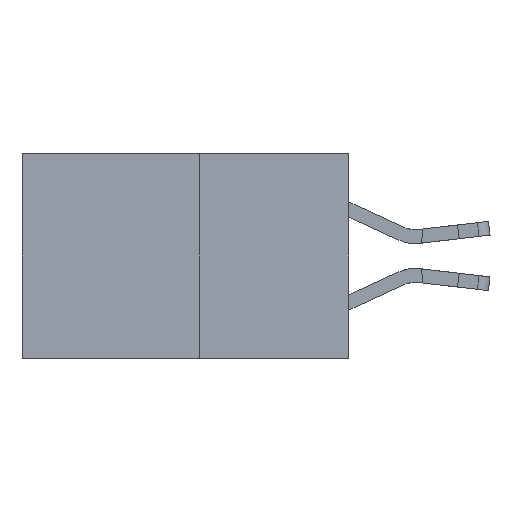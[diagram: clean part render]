
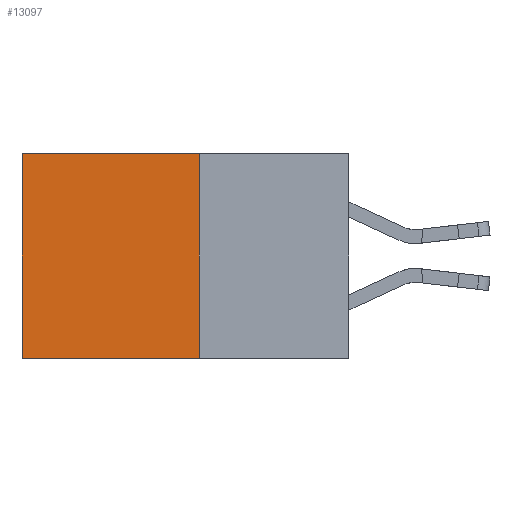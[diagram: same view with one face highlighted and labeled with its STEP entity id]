
A CAD part, left-side view. The second image highlights one B-rep face of the part: STEP entity #13097.
In plain terms, the highlighted planar face has unit normal (-1, 0, 0).
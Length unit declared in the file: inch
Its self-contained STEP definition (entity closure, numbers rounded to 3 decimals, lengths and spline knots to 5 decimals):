
#431 = DIRECTION ( 'NONE',  ( 0., 0., -1. ) ) ;
#689 = EDGE_LOOP ( 'NONE', ( #3078, #10566, #5429, #3585 ) ) ;
#1129 = CARTESIAN_POINT ( 'NONE',  ( 0.277, 0.27, -0.37 ) ) ;
#1178 = EDGE_CURVE ( 'NONE', #10674, #6368, #12203, .T. ) ;
#2004 = CARTESIAN_POINT ( 'NONE',  ( 0.277, 0.59, -0.37 ) ) ;
#2106 = DIRECTION ( 'NONE',  ( 0., 1., 0. ) ) ;
#2155 = LINE ( 'NONE', #2004, #4682 ) ;
#2842 = AXIS2_PLACEMENT_3D ( 'NONE', #1129, #12595, #6492 ) ;
#3014 = CARTESIAN_POINT ( 'NONE',  ( 0.277, 0.27, -0.37 ) ) ;
#3078 = ORIENTED_EDGE ( 'NONE', *, *, #10289, .T. ) ;
#3348 = PLANE ( 'NONE',  #2842 ) ;
#3585 = ORIENTED_EDGE ( 'NONE', *, *, #1178, .T. ) ;
#3649 = VERTEX_POINT ( 'NONE', #10205 ) ;
#4003 = VECTOR ( 'NONE', #6234, 39.37008 ) ;
#4246 = FACE_OUTER_BOUND ( 'NONE', #689, .T. ) ;
#4682 = VECTOR ( 'NONE', #13278, 39.37008 ) ;
#4811 = CARTESIAN_POINT ( 'NONE',  ( 0.277, 0.27, 0. ) ) ;
#5087 = VERTEX_POINT ( 'NONE', #10917 ) ;
#5429 = ORIENTED_EDGE ( 'NONE', *, *, #5829, .F. ) ;
#5443 = EDGE_CURVE ( 'NONE', #5087, #3649, #7518, .T. ) ;
#5736 = LINE ( 'NONE', #8645, #10895 ) ;
#5829 = EDGE_CURVE ( 'NONE', #10674, #5087, #5736, .T. ) ;
#6234 = DIRECTION ( 'NONE',  ( 0., 1., 0. ) ) ;
#6368 = VERTEX_POINT ( 'NONE', #8462 ) ;
#6492 = DIRECTION ( 'NONE',  ( 0., 0., -1. ) ) ;
#7344 = CARTESIAN_POINT ( 'NONE',  ( 0.277, 0.27, 0. ) ) ;
#7518 = LINE ( 'NONE', #3014, #12601 ) ;
#8462 = CARTESIAN_POINT ( 'NONE',  ( 0.277, 0.59, 0. ) ) ;
#8645 = CARTESIAN_POINT ( 'NONE',  ( 0.277, 0.27, -0.37 ) ) ;
#10205 = CARTESIAN_POINT ( 'NONE',  ( 0.277, 0.59, -0.37 ) ) ;
#10289 = EDGE_CURVE ( 'NONE', #6368, #3649, #2155, .T. ) ;
#10566 = ORIENTED_EDGE ( 'NONE', *, *, #5443, .F. ) ;
#10674 = VERTEX_POINT ( 'NONE', #4811 ) ;
#10895 = VECTOR ( 'NONE', #431, 39.37008 ) ;
#10917 = CARTESIAN_POINT ( 'NONE',  ( 0.277, 0.27, -0.37 ) ) ;
#12203 = LINE ( 'NONE', #7344, #4003 ) ;
#12595 = DIRECTION ( 'NONE',  ( 1., 0., 0. ) ) ;
#12601 = VECTOR ( 'NONE', #2106, 39.37008 ) ;
#13097 = ADVANCED_FACE ( 'NONE', ( #4246 ), #3348, .F. ) ;
#13278 = DIRECTION ( 'NONE',  ( 0., 0., -1. ) ) ;
